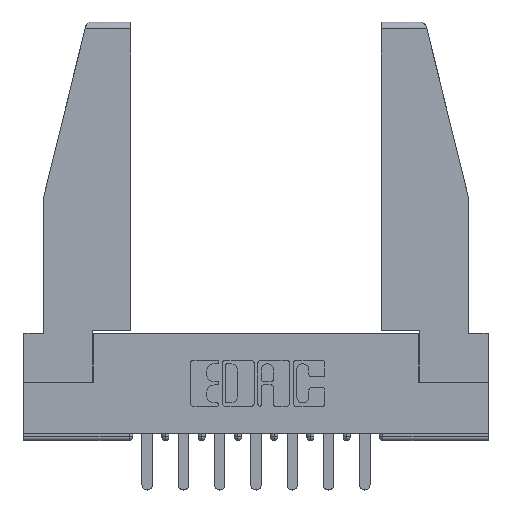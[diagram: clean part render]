
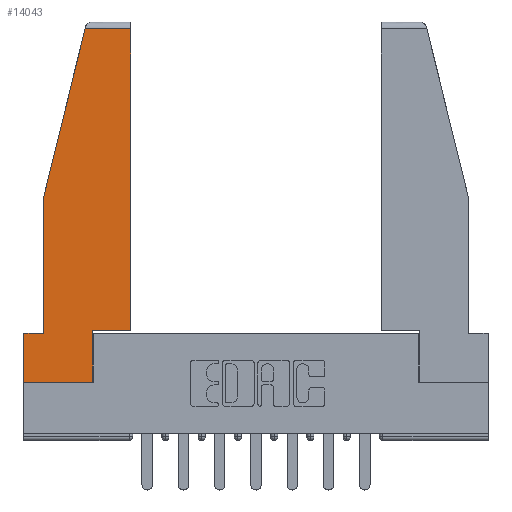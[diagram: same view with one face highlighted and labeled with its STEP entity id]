
A CAD part, top view. The second image highlights one B-rep face of the part: STEP entity #14043.
In plain terms, the highlighted planar face has unit normal (0, 0, 1).
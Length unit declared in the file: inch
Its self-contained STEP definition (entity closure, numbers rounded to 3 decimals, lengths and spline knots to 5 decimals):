
#38 = EDGE_CURVE ( 'NONE', #12565, #6377, #6407, .T. ) ;
#100 = CARTESIAN_POINT ( 'NONE',  ( 0.297, 0., 0. ) ) ;
#127 = EDGE_CURVE ( 'NONE', #2578, #4994, #8975, .T. ) ;
#253 = VECTOR ( 'NONE', #12117, 39.37008 ) ;
#261 = VECTOR ( 'NONE', #4271, 39.37008 ) ;
#274 = CARTESIAN_POINT ( 'NONE',  ( 0., 0.21, 0. ) ) ;
#408 = ORIENTED_EDGE ( 'NONE', *, *, #12661, .T. ) ;
#478 = CARTESIAN_POINT ( 'NONE',  ( 0., 0., 0. ) ) ;
#747 = VECTOR ( 'NONE', #8008, 39.37008 ) ;
#1026 = ORIENTED_EDGE ( 'NONE', *, *, #5646, .T. ) ;
#1160 = CARTESIAN_POINT ( 'NONE',  ( 0., 1.52, 0. ) ) ;
#1182 = EDGE_LOOP ( 'NONE', ( #2056, #9808, #1026, #4270, #1827, #408, #6413, #5629, #8774 ) ) ;
#1423 = VERTEX_POINT ( 'NONE', #8756 ) ;
#1621 = CARTESIAN_POINT ( 'NONE',  ( 0.297, 0.223, 0. ) ) ;
#1827 = ORIENTED_EDGE ( 'NONE', *, *, #4880, .T. ) ;
#1951 = DIRECTION ( 'NONE',  ( 1., 0., 0. ) ) ;
#2011 = CARTESIAN_POINT ( 'NONE',  ( 0.086, 0.8, 0. ) ) ;
#2056 = ORIENTED_EDGE ( 'NONE', *, *, #2408, .T. ) ;
#2399 = EDGE_CURVE ( 'NONE', #4994, #14006, #12126, .T. ) ;
#2408 = EDGE_CURVE ( 'NONE', #14006, #12565, #7003, .T. ) ;
#2578 = VERTEX_POINT ( 'NONE', #100 ) ;
#3715 = CARTESIAN_POINT ( 'NONE',  ( 0.461, 0.223, 0. ) ) ;
#3721 = VERTEX_POINT ( 'NONE', #478 ) ;
#4270 = ORIENTED_EDGE ( 'NONE', *, *, #7205, .T. ) ;
#4271 = DIRECTION ( 'NONE',  ( -1., 0., 0. ) ) ;
#4880 = EDGE_CURVE ( 'NONE', #1423, #10713, #11699, .T. ) ;
#4994 = VERTEX_POINT ( 'NONE', #6080 ) ;
#5161 = DIRECTION ( 'NONE',  ( 0., -1., 0. ) ) ;
#5441 = VECTOR ( 'NONE', #9237, 39.37008 ) ;
#5629 = ORIENTED_EDGE ( 'NONE', *, *, #127, .T. ) ;
#5646 = EDGE_CURVE ( 'NONE', #6377, #12070, #6039, .T. ) ;
#6039 = LINE ( 'NONE', #8526, #9285 ) ;
#6080 = CARTESIAN_POINT ( 'NONE',  ( 0.297, 0.223, 0. ) ) ;
#6294 = VECTOR ( 'NONE', #13646, 39.37008 ) ;
#6355 = CARTESIAN_POINT ( 'NONE',  ( 0.2636, 1.52, 0. ) ) ;
#6377 = VERTEX_POINT ( 'NONE', #6355 ) ;
#6407 = LINE ( 'NONE', #1160, #261 ) ;
#6413 = ORIENTED_EDGE ( 'NONE', *, *, #9016, .T. ) ;
#6476 = VECTOR ( 'NONE', #11623, 39.37008 ) ;
#6894 = CARTESIAN_POINT ( 'NONE',  ( 0.086, 0.8, 0. ) ) ;
#7003 = LINE ( 'NONE', #3715, #6294 ) ;
#7205 = EDGE_CURVE ( 'NONE', #12070, #1423, #9428, .T. ) ;
#7225 = CARTESIAN_POINT ( 'NONE',  ( 0.461, 0.223, 0. ) ) ;
#7540 = CARTESIAN_POINT ( 'NONE',  ( 0., 0., 0. ) ) ;
#7756 = VECTOR ( 'NONE', #11201, 39.37008 ) ;
#7760 = FACE_OUTER_BOUND ( 'NONE', #1182, .T. ) ;
#8008 = DIRECTION ( 'NONE',  ( -1., 0., 0. ) ) ;
#8510 = DIRECTION ( 'NONE',  ( 0., 0., 1. ) ) ;
#8526 = CARTESIAN_POINT ( 'NONE',  ( 0.271, 1.55, 0. ) ) ;
#8756 = CARTESIAN_POINT ( 'NONE',  ( 0.086, 0.21, 0. ) ) ;
#8774 = ORIENTED_EDGE ( 'NONE', *, *, #2399, .T. ) ;
#8975 = LINE ( 'NONE', #10113, #253 ) ;
#9016 = EDGE_CURVE ( 'NONE', #3721, #2578, #9198, .T. ) ;
#9198 = LINE ( 'NONE', #13789, #6476 ) ;
#9237 = DIRECTION ( 'NONE',  ( 1., 0., 0. ) ) ;
#9285 = VECTOR ( 'NONE', #9705, 39.37008 ) ;
#9428 = LINE ( 'NONE', #2011, #12504 ) ;
#9680 = CARTESIAN_POINT ( 'NONE',  ( 0.461, 1.52, 0. ) ) ;
#9705 = DIRECTION ( 'NONE',  ( -0.239, -0.971, 0. ) ) ;
#9808 = ORIENTED_EDGE ( 'NONE', *, *, #38, .T. ) ;
#10080 = CARTESIAN_POINT ( 'NONE',  ( 0., 0.21, 0. ) ) ;
#10113 = CARTESIAN_POINT ( 'NONE',  ( 0.297, 0., 0. ) ) ;
#10153 = CARTESIAN_POINT ( 'NONE',  ( 0., 0.21, 0. ) ) ;
#10441 = AXIS2_PLACEMENT_3D ( 'NONE', #7540, #8510, #1951 ) ;
#10654 = PLANE ( 'NONE',  #10441 ) ;
#10713 = VERTEX_POINT ( 'NONE', #274 ) ;
#11201 = DIRECTION ( 'NONE',  ( 0., -1., 0. ) ) ;
#11623 = DIRECTION ( 'NONE',  ( 1., 0., 0. ) ) ;
#11699 = LINE ( 'NONE', #10153, #747 ) ;
#12070 = VERTEX_POINT ( 'NONE', #6894 ) ;
#12117 = DIRECTION ( 'NONE',  ( 0., 1., 0. ) ) ;
#12126 = LINE ( 'NONE', #1621, #5441 ) ;
#12208 = LINE ( 'NONE', #10080, #7756 ) ;
#12504 = VECTOR ( 'NONE', #5161, 39.37008 ) ;
#12565 = VERTEX_POINT ( 'NONE', #9680 ) ;
#12661 = EDGE_CURVE ( 'NONE', #10713, #3721, #12208, .T. ) ;
#13646 = DIRECTION ( 'NONE',  ( 0., 1., 0. ) ) ;
#13789 = CARTESIAN_POINT ( 'NONE',  ( 0., 0., 0. ) ) ;
#14006 = VERTEX_POINT ( 'NONE', #7225 ) ;
#14043 = ADVANCED_FACE ( 'NONE', ( #7760 ), #10654, .T. ) ;
